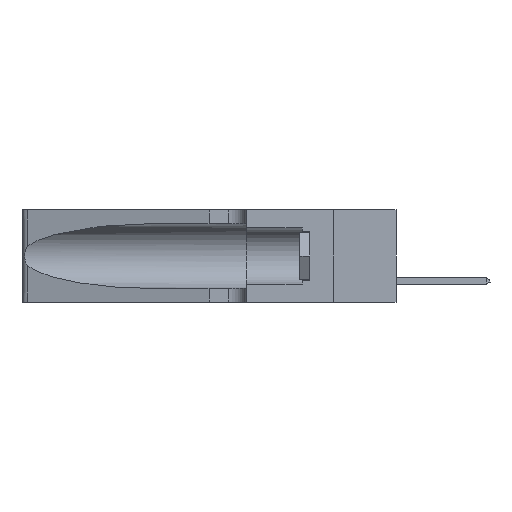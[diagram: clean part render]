
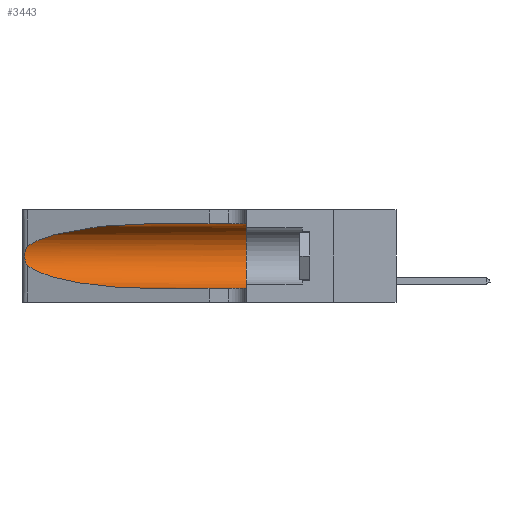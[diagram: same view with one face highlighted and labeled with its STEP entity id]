
A CAD part, left-side view. The second image highlights one B-rep face of the part: STEP entity #3443.
In plain terms, the highlighted cylindrical face has radius 3.308 mm (diameter 6.617 mm), a partial arc.
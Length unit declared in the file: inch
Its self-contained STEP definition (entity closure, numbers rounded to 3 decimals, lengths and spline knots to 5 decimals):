
#188 = CARTESIAN_POINT ( 'NONE',  ( 0.18966, 0.96281, 0.31525 ) ) ;
#660 = CYLINDRICAL_SURFACE ( 'NONE', #11844, 0.13025 ) ;
#908 = EDGE_CURVE ( 'NONE', #973, #16742, #18031, .T. ) ;
#973 = VERTEX_POINT ( 'NONE', #4776 ) ;
#1164 = VERTEX_POINT ( 'NONE', #13845 ) ;
#1337 = CARTESIAN_POINT ( 'NONE',  ( 0.25854, 1.2359, 0.20912 ) ) ;
#1815 = ORIENTED_EDGE ( 'NONE', *, *, #10879, .T. ) ;
#1868 = B_SPLINE_CURVE_WITH_KNOTS ( 'NONE', 3,
 ( #5558, #14994, #6022, #17579, #1337, #14271, #2977, #15819, #11027, #20727, #12677, #4621, #9250, #15892 ),
 .UNSPECIFIED., .F., .F.,
 ( 4, 2, 2, 2, 2, 2, 4 ),
 ( 0., 0.00027, 0.00053, 0.00107, 0.0016, 0.00187, 0.00214 ),
 .UNSPECIFIED. ) ;
#2153 = CARTESIAN_POINT ( 'NONE',  ( 0.25487, 1.22718, 0.22369 ) ) ;
#2301 = VECTOR ( 'NONE', #19434, 39.37008 ) ;
#2977 = CARTESIAN_POINT ( 'NONE',  ( 0.26075, 1.23896, 0.19203 ) ) ;
#3443 = ADVANCED_FACE ( 'NONE', ( #14727 ), #660, .F. ) ;
#4621 = CARTESIAN_POINT ( 'NONE',  ( 0.25639, 1.23186, 0.15144 ) ) ;
#4776 = CARTESIAN_POINT ( 'NONE',  ( 0.25487, 1.22718, 0.14631 ) ) ;
#5223 = CARTESIAN_POINT ( 'NONE',  ( 0.1305, 0.35, 0.185 ) ) ;
#5558 = CARTESIAN_POINT ( 'NONE',  ( 0.25487, 1.22718, 0.22369 ) ) ;
#5700 = EDGE_CURVE ( 'NONE', #1164, #973, #1868, .T. ) ;
#6021 = VERTEX_POINT ( 'NONE', #15468 ) ;
#6022 = CARTESIAN_POINT ( 'NONE',  ( 0.25639, 1.23184, 0.21858 ) ) ;
#6099 = CARTESIAN_POINT ( 'NONE',  ( 0.1305, 0.72297, 0.05475 ) ) ;
#6463 = DIRECTION ( 'NONE',  ( 0., 0., 1. ) ) ;
#6875 = ORIENTED_EDGE ( 'NONE', *, *, #908, .T. ) ;
#8340 = ORIENTED_EDGE ( 'NONE', *, *, #9478, .T. ) ;
#8454 = CARTESIAN_POINT ( 'NONE',  ( 0.1305, 0.35, 0.05475 ) ) ;
#8962 = ORIENTED_EDGE ( 'NONE', *, *, #18340, .F. ) ;
#9250 = CARTESIAN_POINT ( 'NONE',  ( 0.25555, 1.22993, 0.14849 ) ) ;
#9450 = EDGE_CURVE ( 'NONE', #17369, #6021, #13607, .T. ) ;
#9478 = EDGE_CURVE ( 'NONE', #17369, #1164, #11809, .T. ) ;
#9697 = DIRECTION ( 'NONE',  ( 0., 1., 0. ) ) ;
#9790 = CARTESIAN_POINT ( 'NONE',  ( 0.1305, 0.72297, 0.31525 ) ) ;
#10121 = DIRECTION ( 'NONE',  ( 0., 0., -1. ) ) ;
#10879 = EDGE_CURVE ( 'NONE', #16742, #14181, #12535, .T. ) ;
#11027 = CARTESIAN_POINT ( 'NONE',  ( 0.26017, 1.23833, 0.17102 ) ) ;
#11809 =( BOUNDED_CURVE ( )  B_SPLINE_CURVE ( 3, ( #9790, #188, #18306, #2153 ),
 .UNSPECIFIED., .F., .F. ) 
 B_SPLINE_CURVE_WITH_KNOTS ( ( 4, 4 ),
 ( 1.5708, 2.84003 ),
 .UNSPECIFIED. ) 
 CURVE ( )  GEOMETRIC_REPRESENTATION_ITEM ( )  RATIONAL_B_SPLINE_CURVE ( ( 1., 0.87, 0.87, 1. ) ) 
 REPRESENTATION_ITEM ( '' )  );
#11844 = AXIS2_PLACEMENT_3D ( 'NONE', #18157, #16551, #10121 ) ;
#12301 = CIRCLE ( 'NONE', #14465, 0.13025 ) ;
#12535 = LINE ( 'NONE', #12539, #15050 ) ;
#12539 = CARTESIAN_POINT ( 'NONE',  ( 0.1305, 1.61858, 0.05475 ) ) ;
#12614 = ORIENTED_EDGE ( 'NONE', *, *, #9450, .F. ) ;
#12677 = CARTESIAN_POINT ( 'NONE',  ( 0.25789, 1.23486, 0.15765 ) ) ;
#13607 = LINE ( 'NONE', #16360, #2301 ) ;
#13845 = CARTESIAN_POINT ( 'NONE',  ( 0.25487, 1.22718, 0.22369 ) ) ;
#14181 = VERTEX_POINT ( 'NONE', #8454 ) ;
#14271 = CARTESIAN_POINT ( 'NONE',  ( 0.26018, 1.23835, 0.19895 ) ) ;
#14465 = AXIS2_PLACEMENT_3D ( 'NONE', #5223, #9697, #6463 ) ;
#14636 = CARTESIAN_POINT ( 'NONE',  ( 0.25487, 1.22718, 0.14631 ) ) ;
#14727 = FACE_OUTER_BOUND ( 'NONE', #14747, .T. ) ;
#14747 = EDGE_LOOP ( 'NONE', ( #8340, #18606, #6875, #1815, #8962, #12614 ) ) ;
#14994 = CARTESIAN_POINT ( 'NONE',  ( 0.25555, 1.22994, 0.2215 ) ) ;
#15050 = VECTOR ( 'NONE', #15685, 39.37008 ) ;
#15468 = CARTESIAN_POINT ( 'NONE',  ( 0.1305, 0.35, 0.31525 ) ) ;
#15685 = DIRECTION ( 'NONE',  ( 0., -1., 0. ) ) ;
#15819 = CARTESIAN_POINT ( 'NONE',  ( 0.26075, 1.23896, 0.178 ) ) ;
#15892 = CARTESIAN_POINT ( 'NONE',  ( 0.25487, 1.22718, 0.14631 ) ) ;
#16360 = CARTESIAN_POINT ( 'NONE',  ( 0.1305, 1.61858, 0.31525 ) ) ;
#16551 = DIRECTION ( 'NONE',  ( 0., -1., 0. ) ) ;
#16742 = VERTEX_POINT ( 'NONE', #6099 ) ;
#17369 = VERTEX_POINT ( 'NONE', #19800 ) ;
#17579 = CARTESIAN_POINT ( 'NONE',  ( 0.25787, 1.23484, 0.2124 ) ) ;
#17862 = CARTESIAN_POINT ( 'NONE',  ( 0.18966, 0.96281, 0.05475 ) ) ;
#17931 = CARTESIAN_POINT ( 'NONE',  ( 0.2373, 1.15595, 0.08982 ) ) ;
#18031 =( BOUNDED_CURVE ( )  B_SPLINE_CURVE ( 3, ( #14636, #17931, #17862, #19250 ),
 .UNSPECIFIED., .F., .T. ) 
 B_SPLINE_CURVE_WITH_KNOTS ( ( 4, 4 ),
 ( 3.44316, 4.71239 ),
 .UNSPECIFIED. ) 
 CURVE ( )  GEOMETRIC_REPRESENTATION_ITEM ( )  RATIONAL_B_SPLINE_CURVE ( ( 1., 0.87, 0.87, 1. ) ) 
 REPRESENTATION_ITEM ( '' )  );
#18157 = CARTESIAN_POINT ( 'NONE',  ( 0.1305, 1.61858, 0.185 ) ) ;
#18306 = CARTESIAN_POINT ( 'NONE',  ( 0.2373, 1.15595, 0.28018 ) ) ;
#18340 = EDGE_CURVE ( 'NONE', #6021, #14181, #12301, .T. ) ;
#18606 = ORIENTED_EDGE ( 'NONE', *, *, #5700, .T. ) ;
#19250 = CARTESIAN_POINT ( 'NONE',  ( 0.1305, 0.72297, 0.05475 ) ) ;
#19434 = DIRECTION ( 'NONE',  ( 0., -1., 0. ) ) ;
#19800 = CARTESIAN_POINT ( 'NONE',  ( 0.1305, 0.72297, 0.31525 ) ) ;
#20727 = CARTESIAN_POINT ( 'NONE',  ( 0.25856, 1.23593, 0.16098 ) ) ;
